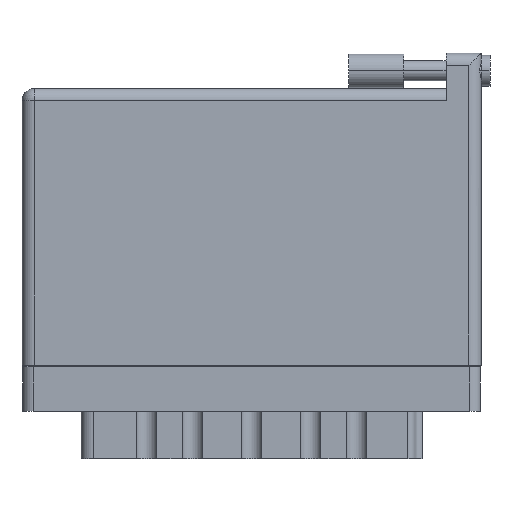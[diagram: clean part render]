
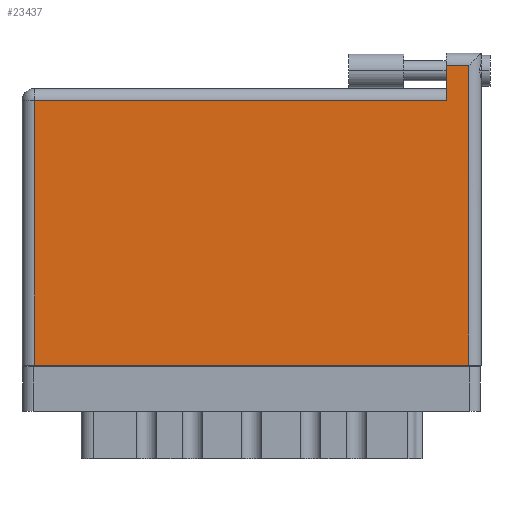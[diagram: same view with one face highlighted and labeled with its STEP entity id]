
A CAD part, front view. The second image highlights one B-rep face of the part: STEP entity #23437.
In plain terms, the highlighted face is planar.
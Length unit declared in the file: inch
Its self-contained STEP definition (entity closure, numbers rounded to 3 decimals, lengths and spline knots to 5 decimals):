
#142 = CARTESIAN_POINT ( 'NONE',  ( 0., 1.696, 0. ) ) ;
#1239 = VECTOR ( 'NONE', #19530, 39.37008 ) ;
#1357 = PLANE ( 'NONE',  #43313 ) ;
#1886 = ORIENTED_EDGE ( 'NONE', *, *, #39275, .T. ) ;
#2648 = DIRECTION ( 'NONE',  ( -1., 0., 0. ) ) ;
#2794 = EDGE_CURVE ( 'NONE', #41732, #36413, #28009, .T. ) ;
#3934 = CARTESIAN_POINT ( 'NONE',  ( 0., 0., 0. ) ) ;
#4569 = VECTOR ( 'NONE', #34352, 39.37008 ) ;
#4880 = EDGE_CURVE ( 'NONE', #14956, #34178, #19413, .T. ) ;
#7976 = CARTESIAN_POINT ( 'NONE',  ( 2.403, 1.496, 0. ) ) ;
#8239 = EDGE_CURVE ( 'NONE', #35883, #10819, #34008, .T. ) ;
#9024 = CARTESIAN_POINT ( 'NONE',  ( 0., 1.566, 0. ) ) ;
#10140 = CARTESIAN_POINT ( 'NONE',  ( 2.53, 0., 0. ) ) ;
#10819 = VERTEX_POINT ( 'NONE', #20197 ) ;
#11801 = DIRECTION ( 'NONE',  ( 0., -1., 0. ) ) ;
#13631 = CARTESIAN_POINT ( 'NONE',  ( 0., 1.496, 0. ) ) ;
#14881 = CARTESIAN_POINT ( 'NONE',  ( 2.403, 1.696, 0. ) ) ;
#14956 = VERTEX_POINT ( 'NONE', #10140 ) ;
#15457 = CARTESIAN_POINT ( 'NONE',  ( 0.07, 0., 0. ) ) ;
#15914 = VECTOR ( 'NONE', #2648, 39.37008 ) ;
#17927 = CARTESIAN_POINT ( 'NONE',  ( 2.403, 1.766, 0. ) ) ;
#18466 = VECTOR ( 'NONE', #11801, 39.37008 ) ;
#19413 = LINE ( 'NONE', #26654, #4569 ) ;
#19530 = DIRECTION ( 'NONE',  ( 1., 0., 0. ) ) ;
#20197 = CARTESIAN_POINT ( 'NONE',  ( 0.07, 0., 0. ) ) ;
#20216 = VECTOR ( 'NONE', #25596, 39.37008 ) ;
#21064 = EDGE_CURVE ( 'NONE', #34178, #41732, #32576, .T. ) ;
#22228 = EDGE_LOOP ( 'NONE', ( #48055, #25164, #29813, #25461, #1886, #46014 ) ) ;
#23437 = ADVANCED_FACE ( 'NONE', ( #49008 ), #1357, .F. ) ;
#23644 = LINE ( 'NONE', #13631, #15914 ) ;
#25164 = ORIENTED_EDGE ( 'NONE', *, *, #4880, .T. ) ;
#25461 = ORIENTED_EDGE ( 'NONE', *, *, #2794, .T. ) ;
#25596 = DIRECTION ( 'NONE',  ( 0., -1., 0. ) ) ;
#26654 = CARTESIAN_POINT ( 'NONE',  ( 2.53, 1.766, 0. ) ) ;
#26770 = DIRECTION ( 'NONE',  ( -1., 0., 0. ) ) ;
#28009 = LINE ( 'NONE', #17927, #20216 ) ;
#28464 = EDGE_CURVE ( 'NONE', #10819, #14956, #41831, .T. ) ;
#29813 = ORIENTED_EDGE ( 'NONE', *, *, #21064, .T. ) ;
#31528 = DIRECTION ( 'NONE',  ( 0., 0., -1. ) ) ;
#32576 = LINE ( 'NONE', #142, #40340 ) ;
#34008 = LINE ( 'NONE', #15457, #18466 ) ;
#34178 = VERTEX_POINT ( 'NONE', #47566 ) ;
#34352 = DIRECTION ( 'NONE',  ( 0., 1., 0. ) ) ;
#35883 = VERTEX_POINT ( 'NONE', #39355 ) ;
#36413 = VERTEX_POINT ( 'NONE', #7976 ) ;
#39275 = EDGE_CURVE ( 'NONE', #36413, #35883, #23644, .T. ) ;
#39355 = CARTESIAN_POINT ( 'NONE',  ( 0.07, 1.496, 0. ) ) ;
#40340 = VECTOR ( 'NONE', #26770, 39.37008 ) ;
#41732 = VERTEX_POINT ( 'NONE', #14881 ) ;
#41831 = LINE ( 'NONE', #3934, #1239 ) ;
#43035 = DIRECTION ( 'NONE',  ( -1., 0., 0. ) ) ;
#43313 = AXIS2_PLACEMENT_3D ( 'NONE', #9024, #31528, #43035 ) ;
#46014 = ORIENTED_EDGE ( 'NONE', *, *, #8239, .T. ) ;
#47566 = CARTESIAN_POINT ( 'NONE',  ( 2.53, 1.696, 0. ) ) ;
#48055 = ORIENTED_EDGE ( 'NONE', *, *, #28464, .T. ) ;
#49008 = FACE_OUTER_BOUND ( 'NONE', #22228, .T. ) ;
